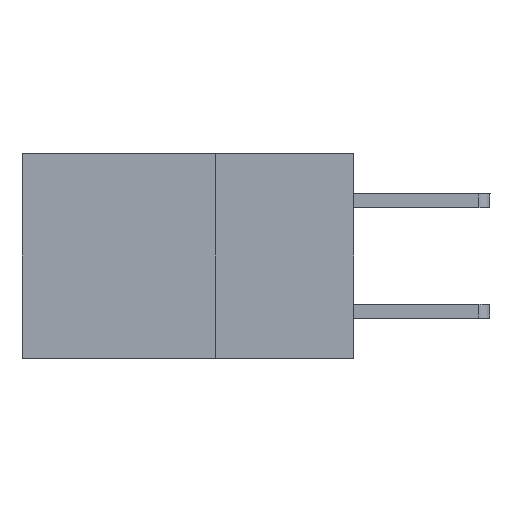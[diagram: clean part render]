
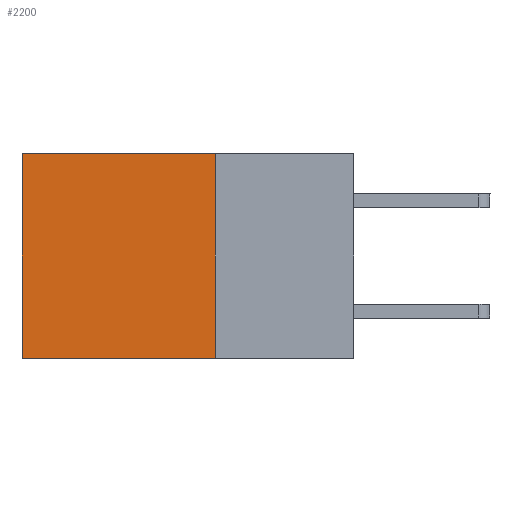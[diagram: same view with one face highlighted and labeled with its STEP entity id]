
A CAD part, left-side view. The second image highlights one B-rep face of the part: STEP entity #2200.
In plain terms, the highlighted planar face has unit normal (-1, 0, 0).
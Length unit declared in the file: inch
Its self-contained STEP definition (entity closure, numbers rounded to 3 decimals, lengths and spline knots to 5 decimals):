
#215 = LINE ( 'NONE', #8738, #11179 ) ;
#578 = EDGE_CURVE ( 'NONE', #1311, #3658, #1587, .T. ) ;
#825 = VECTOR ( 'NONE', #12795, 39.37008 ) ;
#1311 = VERTEX_POINT ( 'NONE', #8509 ) ;
#1587 = LINE ( 'NONE', #4440, #9683 ) ;
#2200 = ADVANCED_FACE ( 'NONE', ( #7051 ), #3586, .F. ) ;
#2438 = DIRECTION ( 'NONE',  ( 0., 1., 0. ) ) ;
#2535 = CARTESIAN_POINT ( 'NONE',  ( 0.2875, 0.25, 0. ) ) ;
#2654 = EDGE_LOOP ( 'NONE', ( #11183, #3547, #8991, #3872 ) ) ;
#2833 = CARTESIAN_POINT ( 'NONE',  ( 0.2875, 0.6, -0.37 ) ) ;
#3350 = DIRECTION ( 'NONE',  ( 0., 0., -1. ) ) ;
#3403 = DIRECTION ( 'NONE',  ( 1., 0., 0. ) ) ;
#3540 = VECTOR ( 'NONE', #2438, 39.37008 ) ;
#3547 = ORIENTED_EDGE ( 'NONE', *, *, #578, .F. ) ;
#3586 = PLANE ( 'NONE',  #9482 ) ;
#3623 = DIRECTION ( 'NONE',  ( 0., 0., -1. ) ) ;
#3658 = VERTEX_POINT ( 'NONE', #2833 ) ;
#3768 = CARTESIAN_POINT ( 'NONE',  ( 0.2875, 0.25, 0. ) ) ;
#3872 = ORIENTED_EDGE ( 'NONE', *, *, #6186, .T. ) ;
#4329 = LINE ( 'NONE', #11867, #825 ) ;
#4440 = CARTESIAN_POINT ( 'NONE',  ( 0.2875, 0.25, -0.37 ) ) ;
#6163 = EDGE_CURVE ( 'NONE', #11797, #3658, #215, .T. ) ;
#6186 = EDGE_CURVE ( 'NONE', #7150, #11797, #8987, .T. ) ;
#7051 = FACE_OUTER_BOUND ( 'NONE', #2654, .T. ) ;
#7150 = VERTEX_POINT ( 'NONE', #2535 ) ;
#8509 = CARTESIAN_POINT ( 'NONE',  ( 0.2875, 0.25, -0.37 ) ) ;
#8536 = DIRECTION ( 'NONE',  ( 0., 1., 0. ) ) ;
#8738 = CARTESIAN_POINT ( 'NONE',  ( 0.2875, 0.6, 0. ) ) ;
#8987 = LINE ( 'NONE', #10648, #3540 ) ;
#8991 = ORIENTED_EDGE ( 'NONE', *, *, #11031, .F. ) ;
#9482 = AXIS2_PLACEMENT_3D ( 'NONE', #3768, #3403, #3350 ) ;
#9683 = VECTOR ( 'NONE', #8536, 39.37008 ) ;
#9944 = CARTESIAN_POINT ( 'NONE',  ( 0.2875, 0.6, 0. ) ) ;
#10648 = CARTESIAN_POINT ( 'NONE',  ( 0.2875, 0.25, 0. ) ) ;
#11031 = EDGE_CURVE ( 'NONE', #7150, #1311, #4329, .T. ) ;
#11179 = VECTOR ( 'NONE', #3623, 39.37008 ) ;
#11183 = ORIENTED_EDGE ( 'NONE', *, *, #6163, .T. ) ;
#11797 = VERTEX_POINT ( 'NONE', #9944 ) ;
#11867 = CARTESIAN_POINT ( 'NONE',  ( 0.2875, 0.25, 0. ) ) ;
#12795 = DIRECTION ( 'NONE',  ( 0., 0., -1. ) ) ;
